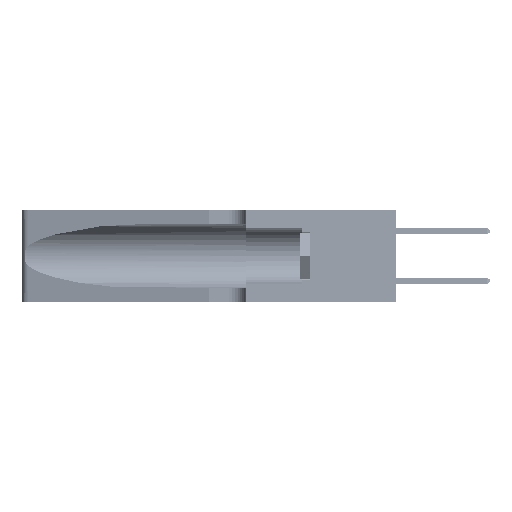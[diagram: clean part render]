
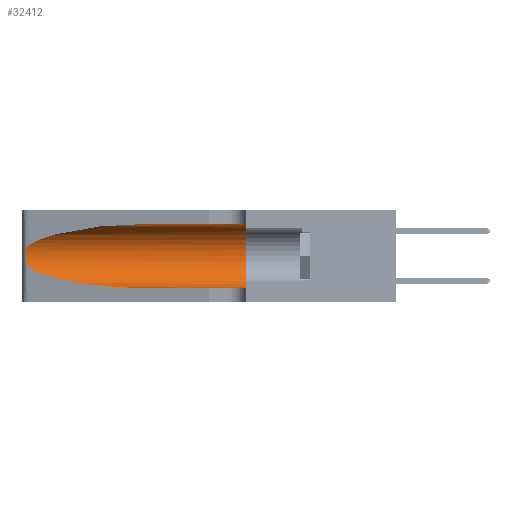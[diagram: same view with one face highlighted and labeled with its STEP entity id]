
A CAD part, left-side view. The second image highlights one B-rep face of the part: STEP entity #32412.
In plain terms, the highlighted cylindrical face has radius 3.308 mm (diameter 6.617 mm), a partial arc.
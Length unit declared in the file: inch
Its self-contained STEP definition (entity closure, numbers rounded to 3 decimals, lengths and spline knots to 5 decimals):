
#117 = CARTESIAN_POINT ( 'NONE',  ( 0.1305, 0.35, 0.05475 ) ) ;
#151 = AXIS2_PLACEMENT_3D ( 'NONE', #12631, #43229, #20493 ) ;
#3473 = CARTESIAN_POINT ( 'NONE',  ( 0.25487, 1.22718, 0.22369 ) ) ;
#3675 = CARTESIAN_POINT ( 'NONE',  ( 0.25487, 1.22718, 0.14631 ) ) ;
#5998 = CARTESIAN_POINT ( 'NONE',  ( 0.25487, 1.22718, 0.22369 ) ) ;
#6403 = CARTESIAN_POINT ( 'NONE',  ( 0.1305, 0.72297, 0.31525 ) ) ;
#6792 = AXIS2_PLACEMENT_3D ( 'NONE', #11271, #37934, #15144 ) ;
#7378 = CARTESIAN_POINT ( 'NONE',  ( 0.25487, 1.22718, 0.22369 ) ) ;
#7466 = EDGE_CURVE ( 'NONE', #23742, #34812, #13664, .T. ) ;
#7604 = VERTEX_POINT ( 'NONE', #23328 ) ;
#8079 = ORIENTED_EDGE ( 'NONE', *, *, #27336, .F. ) ;
#9040 = CYLINDRICAL_SURFACE ( 'NONE', #151, 0.13025 ) ;
#9940 =( BOUNDED_CURVE ( )  B_SPLINE_CURVE ( 3, ( #22623, #15099, #45515, #22786 ),
 .UNSPECIFIED., .F., .F. ) 
 B_SPLINE_CURVE_WITH_KNOTS ( ( 4, 4 ),
 ( 3.44316, 4.71239 ),
 .UNSPECIFIED. ) 
 CURVE ( )  GEOMETRIC_REPRESENTATION_ITEM ( )  RATIONAL_B_SPLINE_CURVE ( ( 1., 0.87, 0.87, 1. ) ) 
 REPRESENTATION_ITEM ( '' )  );
#11169 = VECTOR ( 'NONE', #28973, 39.37008 ) ;
#11271 = CARTESIAN_POINT ( 'NONE',  ( 0.1305, 0.35, 0.185 ) ) ;
#11280 = CARTESIAN_POINT ( 'NONE',  ( 0.25854, 1.2359, 0.20912 ) ) ;
#12631 = CARTESIAN_POINT ( 'NONE',  ( 0.1305, 1.61858, 0.185 ) ) ;
#13664 = B_SPLINE_CURVE_WITH_KNOTS ( 'NONE', 3,
 ( #7378, #30293, #45401, #34135, #11280, #37940, #15153, #41755, #19020, #45566, #22833, #49388, #26651, #3675 ),
 .UNSPECIFIED., .F., .F.,
 ( 4, 2, 2, 2, 2, 2, 4 ),
 ( 0., 0.00027, 0.00053, 0.00107, 0.0016, 0.00187, 0.00214 ),
 .UNSPECIFIED. ) ;
#14511 = VERTEX_POINT ( 'NONE', #6403 ) ;
#15099 = CARTESIAN_POINT ( 'NONE',  ( 0.2373, 1.15595, 0.08982 ) ) ;
#15144 = DIRECTION ( 'NONE',  ( 0., 0., 1. ) ) ;
#15153 = CARTESIAN_POINT ( 'NONE',  ( 0.26075, 1.23896, 0.19203 ) ) ;
#17494 = CARTESIAN_POINT ( 'NONE',  ( 0.1305, 0.72297, 0.31525 ) ) ;
#18541 = EDGE_CURVE ( 'NONE', #7604, #46078, #46464, .T. ) ;
#18882 =( BOUNDED_CURVE ( )  B_SPLINE_CURVE ( 3, ( #17494, #44047, #28938, #5998 ),
 .UNSPECIFIED., .F., .T. ) 
 B_SPLINE_CURVE_WITH_KNOTS ( ( 4, 4 ),
 ( 1.5708, 2.84003 ),
 .UNSPECIFIED. ) 
 CURVE ( )  GEOMETRIC_REPRESENTATION_ITEM ( )  RATIONAL_B_SPLINE_CURVE ( ( 1., 0.87, 0.87, 1. ) ) 
 REPRESENTATION_ITEM ( '' )  );
#19020 = CARTESIAN_POINT ( 'NONE',  ( 0.26017, 1.23833, 0.17102 ) ) ;
#20021 = EDGE_CURVE ( 'NONE', #14511, #31300, #21383, .T. ) ;
#20493 = DIRECTION ( 'NONE',  ( 0., 0., -1. ) ) ;
#20708 = ORIENTED_EDGE ( 'NONE', *, *, #18541, .T. ) ;
#20837 = DIRECTION ( 'NONE',  ( 0., -1., 0. ) ) ;
#21362 = CARTESIAN_POINT ( 'NONE',  ( 0.1305, 1.61858, 0.31525 ) ) ;
#21383 = LINE ( 'NONE', #21362, #11169 ) ;
#21754 = CARTESIAN_POINT ( 'NONE',  ( 0.1305, 0.35, 0.31525 ) ) ;
#22623 = CARTESIAN_POINT ( 'NONE',  ( 0.25487, 1.22718, 0.14631 ) ) ;
#22786 = CARTESIAN_POINT ( 'NONE',  ( 0.1305, 0.72297, 0.05475 ) ) ;
#22833 = CARTESIAN_POINT ( 'NONE',  ( 0.25789, 1.23486, 0.15765 ) ) ;
#23328 = CARTESIAN_POINT ( 'NONE',  ( 0.1305, 0.72297, 0.05475 ) ) ;
#23742 = VERTEX_POINT ( 'NONE', #3473 ) ;
#24633 = CARTESIAN_POINT ( 'NONE',  ( 0.1305, 1.61858, 0.05475 ) ) ;
#26275 = VECTOR ( 'NONE', #20837, 39.37008 ) ;
#26651 = CARTESIAN_POINT ( 'NONE',  ( 0.25555, 1.22993, 0.14849 ) ) ;
#27336 = EDGE_CURVE ( 'NONE', #31300, #46078, #33107, .T. ) ;
#27617 = ORIENTED_EDGE ( 'NONE', *, *, #7466, .T. ) ;
#28938 = CARTESIAN_POINT ( 'NONE',  ( 0.2373, 1.15595, 0.28018 ) ) ;
#28973 = DIRECTION ( 'NONE',  ( 0., -1., 0. ) ) ;
#30161 = EDGE_CURVE ( 'NONE', #14511, #23742, #18882, .T. ) ;
#30293 = CARTESIAN_POINT ( 'NONE',  ( 0.25555, 1.22994, 0.2215 ) ) ;
#31300 = VERTEX_POINT ( 'NONE', #21754 ) ;
#32412 = ADVANCED_FACE ( 'NONE', ( #41862 ), #9040, .F. ) ;
#32800 = EDGE_CURVE ( 'NONE', #34812, #7604, #9940, .T. ) ;
#33107 = CIRCLE ( 'NONE', #6792, 0.13025 ) ;
#34135 = CARTESIAN_POINT ( 'NONE',  ( 0.25787, 1.23484, 0.2124 ) ) ;
#34606 = ORIENTED_EDGE ( 'NONE', *, *, #20021, .F. ) ;
#34812 = VERTEX_POINT ( 'NONE', #41561 ) ;
#36866 = ORIENTED_EDGE ( 'NONE', *, *, #30161, .T. ) ;
#37934 = DIRECTION ( 'NONE',  ( 0., 1., 0. ) ) ;
#37940 = CARTESIAN_POINT ( 'NONE',  ( 0.26018, 1.23835, 0.19895 ) ) ;
#41561 = CARTESIAN_POINT ( 'NONE',  ( 0.25487, 1.22718, 0.14631 ) ) ;
#41755 = CARTESIAN_POINT ( 'NONE',  ( 0.26075, 1.23896, 0.178 ) ) ;
#41862 = FACE_OUTER_BOUND ( 'NONE', #45057, .T. ) ;
#43229 = DIRECTION ( 'NONE',  ( 0., -1., 0. ) ) ;
#44047 = CARTESIAN_POINT ( 'NONE',  ( 0.18966, 0.96281, 0.31525 ) ) ;
#45057 = EDGE_LOOP ( 'NONE', ( #36866, #27617, #47789, #20708, #8079, #34606 ) ) ;
#45401 = CARTESIAN_POINT ( 'NONE',  ( 0.25639, 1.23184, 0.21858 ) ) ;
#45515 = CARTESIAN_POINT ( 'NONE',  ( 0.18966, 0.96281, 0.05475 ) ) ;
#45566 = CARTESIAN_POINT ( 'NONE',  ( 0.25856, 1.23593, 0.16098 ) ) ;
#46078 = VERTEX_POINT ( 'NONE', #117 ) ;
#46464 = LINE ( 'NONE', #24633, #26275 ) ;
#47789 = ORIENTED_EDGE ( 'NONE', *, *, #32800, .T. ) ;
#49388 = CARTESIAN_POINT ( 'NONE',  ( 0.25639, 1.23186, 0.15144 ) ) ;
